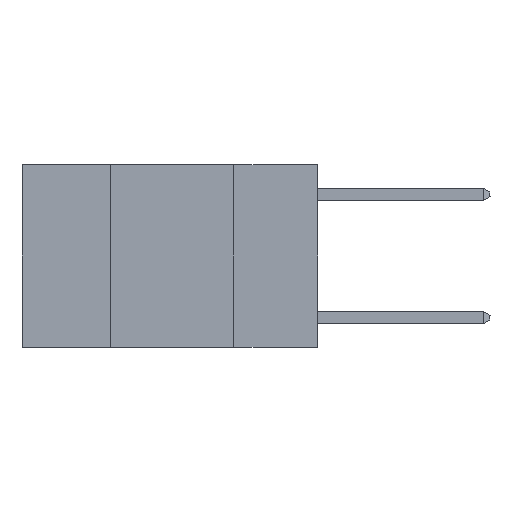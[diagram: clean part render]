
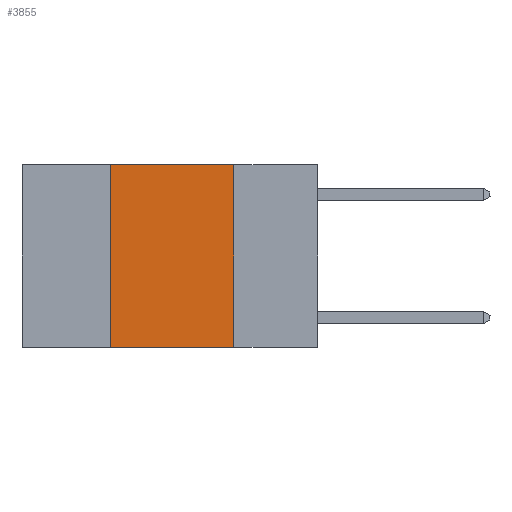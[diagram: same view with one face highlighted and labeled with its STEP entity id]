
A CAD part, left-side view. The second image highlights one B-rep face of the part: STEP entity #3855.
In plain terms, the highlighted planar face has unit normal (-1, 0, 0).
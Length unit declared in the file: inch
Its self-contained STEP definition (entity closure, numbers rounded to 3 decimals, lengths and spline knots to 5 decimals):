
#58 = VERTEX_POINT ( 'NONE', #3404 ) ;
#517 = EDGE_CURVE ( 'NONE', #7138, #21556, #24464, .T. ) ;
#3404 = CARTESIAN_POINT ( 'NONE',  ( 0., 0.17, 0. ) ) ;
#3855 = ADVANCED_FACE ( 'NONE', ( #4351 ), #23186, .F. ) ;
#4351 = FACE_OUTER_BOUND ( 'NONE', #13539, .T. ) ;
#4606 = EDGE_CURVE ( 'NONE', #7138, #7705, #16682, .T. ) ;
#4770 = DIRECTION ( 'NONE',  ( 0., 0., -1. ) ) ;
#7138 = VERTEX_POINT ( 'NONE', #24321 ) ;
#7236 = VECTOR ( 'NONE', #18309, 39.37008 ) ;
#7576 = VECTOR ( 'NONE', #23168, 39.37008 ) ;
#7705 = VERTEX_POINT ( 'NONE', #23092 ) ;
#8820 = LINE ( 'NONE', #18888, #22645 ) ;
#8872 = ORIENTED_EDGE ( 'NONE', *, *, #14983, .F. ) ;
#11325 = AXIS2_PLACEMENT_3D ( 'NONE', #16897, #25423, #4770 ) ;
#11552 = ORIENTED_EDGE ( 'NONE', *, *, #4606, .T. ) ;
#11930 = CARTESIAN_POINT ( 'NONE',  ( 0., 0.42, 0. ) ) ;
#12168 = EDGE_CURVE ( 'NONE', #21556, #58, #8820, .T. ) ;
#12413 = LINE ( 'NONE', #21368, #7576 ) ;
#13539 = EDGE_LOOP ( 'NONE', ( #8872, #17538, #17386, #11552 ) ) ;
#14579 = DIRECTION ( 'NONE',  ( 0., -1., 0. ) ) ;
#14677 = DIRECTION ( 'NONE',  ( 0., -1., 0. ) ) ;
#14983 = EDGE_CURVE ( 'NONE', #58, #7705, #12413, .T. ) ;
#15606 = VECTOR ( 'NONE', #14579, 39.37008 ) ;
#16682 = LINE ( 'NONE', #25072, #15606 ) ;
#16897 = CARTESIAN_POINT ( 'NONE',  ( 0., 0.6, 0. ) ) ;
#17386 = ORIENTED_EDGE ( 'NONE', *, *, #517, .F. ) ;
#17538 = ORIENTED_EDGE ( 'NONE', *, *, #12168, .F. ) ;
#18309 = DIRECTION ( 'NONE',  ( 0., 0., 1. ) ) ;
#18888 = CARTESIAN_POINT ( 'NONE',  ( 0., 0.6, 0. ) ) ;
#21368 = CARTESIAN_POINT ( 'NONE',  ( 0., 0.17, 0. ) ) ;
#21556 = VERTEX_POINT ( 'NONE', #11930 ) ;
#22645 = VECTOR ( 'NONE', #14677, 39.37008 ) ;
#23092 = CARTESIAN_POINT ( 'NONE',  ( 0., 0.17, -0.37 ) ) ;
#23168 = DIRECTION ( 'NONE',  ( 0., 0., -1. ) ) ;
#23186 = PLANE ( 'NONE',  #11325 ) ;
#24321 = CARTESIAN_POINT ( 'NONE',  ( 0., 0.42, -0.37 ) ) ;
#24333 = CARTESIAN_POINT ( 'NONE',  ( 0., 0.42, 0. ) ) ;
#24464 = LINE ( 'NONE', #24333, #7236 ) ;
#25072 = CARTESIAN_POINT ( 'NONE',  ( 0., 0.6, -0.37 ) ) ;
#25423 = DIRECTION ( 'NONE',  ( 1., 0., 0. ) ) ;
